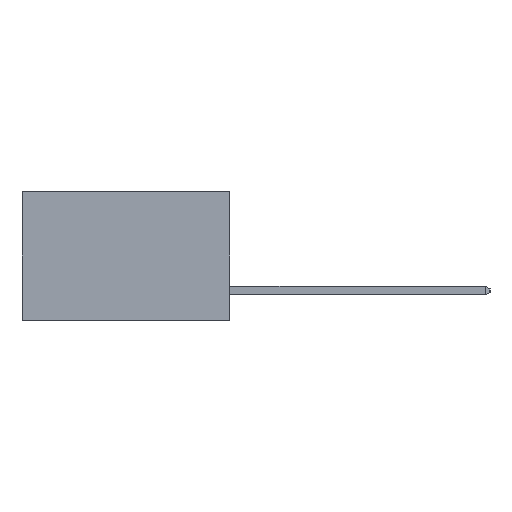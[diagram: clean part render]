
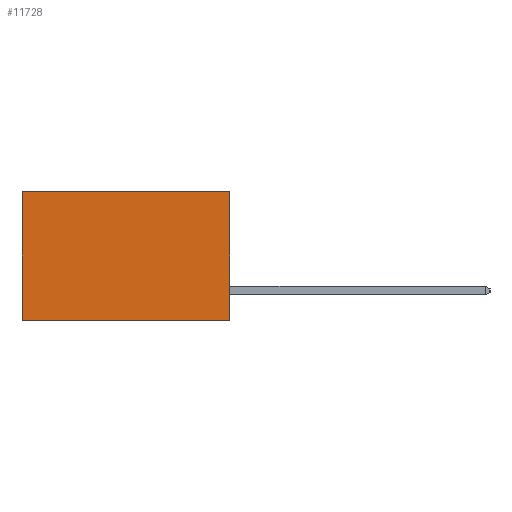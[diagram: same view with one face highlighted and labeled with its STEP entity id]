
A CAD part, left-side view. The second image highlights one B-rep face of the part: STEP entity #11728.
In plain terms, the highlighted planar face has unit normal (-1, 0, 0).
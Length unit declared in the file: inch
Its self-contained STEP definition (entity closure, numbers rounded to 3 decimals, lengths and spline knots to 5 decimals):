
#1134 = VECTOR ( 'NONE', #12609, 39.37008 ) ;
#3582 = ORIENTED_EDGE ( 'NONE', *, *, #3840, .F. ) ;
#3840 = EDGE_CURVE ( 'NONE', #11725, #8922, #12435, .T. ) ;
#4513 = CARTESIAN_POINT ( 'NONE',  ( 0.298, 0., 0. ) ) ;
#4697 = CARTESIAN_POINT ( 'NONE',  ( 0.298, 0., -0.37 ) ) ;
#5439 = LINE ( 'NONE', #21888, #9842 ) ;
#6838 = CARTESIAN_POINT ( 'NONE',  ( 0.298, 0., 0. ) ) ;
#6885 = VECTOR ( 'NONE', #10219, 39.37008 ) ;
#7601 = CARTESIAN_POINT ( 'NONE',  ( 0.298, 0.6, 0. ) ) ;
#8154 = CARTESIAN_POINT ( 'NONE',  ( 0.298, 0.6, -0.37 ) ) ;
#8318 = DIRECTION ( 'NONE',  ( 0., 0., -1. ) ) ;
#8376 = EDGE_CURVE ( 'NONE', #19514, #8922, #11843, .T. ) ;
#8478 = ORIENTED_EDGE ( 'NONE', *, *, #22360, .T. ) ;
#8922 = VERTEX_POINT ( 'NONE', #8154 ) ;
#9094 = VERTEX_POINT ( 'NONE', #6838 ) ;
#9530 = EDGE_LOOP ( 'NONE', ( #19252, #3582, #14784, #8478 ) ) ;
#9842 = VECTOR ( 'NONE', #14697, 39.37008 ) ;
#10030 = PLANE ( 'NONE',  #22671 ) ;
#10219 = DIRECTION ( 'NONE',  ( 0., 0., -1. ) ) ;
#10755 = CARTESIAN_POINT ( 'NONE',  ( 0.298, 0., 0. ) ) ;
#11254 = LINE ( 'NONE', #10755, #1134 ) ;
#11725 = VERTEX_POINT ( 'NONE', #15652 ) ;
#11728 = ADVANCED_FACE ( 'NONE', ( #23018 ), #10030, .F. ) ;
#11843 = LINE ( 'NONE', #21134, #6885 ) ;
#12435 = LINE ( 'NONE', #4697, #19236 ) ;
#12609 = DIRECTION ( 'NONE',  ( 0., 0., -1. ) ) ;
#14320 = EDGE_CURVE ( 'NONE', #9094, #11725, #11254, .T. ) ;
#14697 = DIRECTION ( 'NONE',  ( 0., 1., 0. ) ) ;
#14784 = ORIENTED_EDGE ( 'NONE', *, *, #14320, .F. ) ;
#15652 = CARTESIAN_POINT ( 'NONE',  ( 0.298, 0., -0.37 ) ) ;
#19236 = VECTOR ( 'NONE', #23594, 39.37008 ) ;
#19252 = ORIENTED_EDGE ( 'NONE', *, *, #8376, .T. ) ;
#19261 = DIRECTION ( 'NONE',  ( 1., 0., 0. ) ) ;
#19514 = VERTEX_POINT ( 'NONE', #7601 ) ;
#21134 = CARTESIAN_POINT ( 'NONE',  ( 0.298, 0.6, 0. ) ) ;
#21888 = CARTESIAN_POINT ( 'NONE',  ( 0.298, 0., 0. ) ) ;
#22360 = EDGE_CURVE ( 'NONE', #9094, #19514, #5439, .T. ) ;
#22671 = AXIS2_PLACEMENT_3D ( 'NONE', #4513, #19261, #8318 ) ;
#23018 = FACE_OUTER_BOUND ( 'NONE', #9530, .T. ) ;
#23594 = DIRECTION ( 'NONE',  ( 0., 1., 0. ) ) ;
